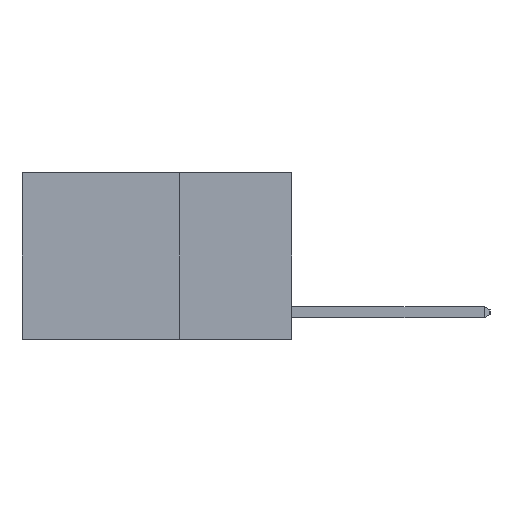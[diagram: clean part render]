
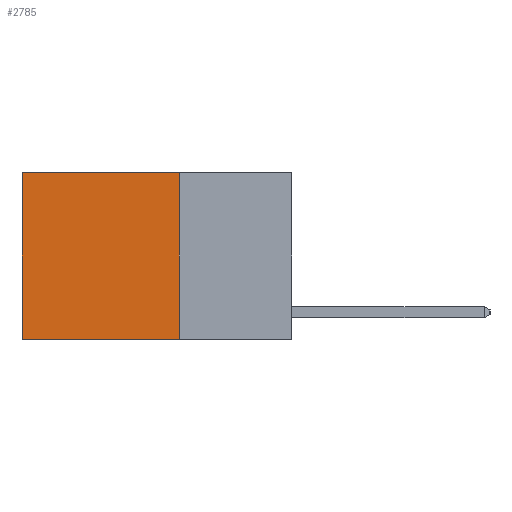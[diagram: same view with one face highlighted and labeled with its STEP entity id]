
A CAD part, left-side view. The second image highlights one B-rep face of the part: STEP entity #2785.
In plain terms, the highlighted planar face has unit normal (-1, 0, 0).
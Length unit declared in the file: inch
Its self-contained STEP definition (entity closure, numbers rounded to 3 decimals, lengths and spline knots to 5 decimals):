
#176 = EDGE_CURVE ( 'NONE', #11325, #1488, #7365, .T. ) ;
#325 = CARTESIAN_POINT ( 'NONE',  ( 0.2625, 0.25, -0.37 ) ) ;
#574 = EDGE_LOOP ( 'NONE', ( #7334, #2866, #12670, #5633 ) ) ;
#580 = EDGE_CURVE ( 'NONE', #3494, #11325, #13664, .T. ) ;
#937 = DIRECTION ( 'NONE',  ( 0., 1., 0. ) ) ;
#1488 = VERTEX_POINT ( 'NONE', #12290 ) ;
#2056 = VERTEX_POINT ( 'NONE', #325 ) ;
#2294 = DIRECTION ( 'NONE',  ( 0., 0., -1. ) ) ;
#2459 = LINE ( 'NONE', #8184, #11899 ) ;
#2785 = ADVANCED_FACE ( 'NONE', ( #12186 ), #4285, .F. ) ;
#2866 = ORIENTED_EDGE ( 'NONE', *, *, #13939, .F. ) ;
#3155 = CARTESIAN_POINT ( 'NONE',  ( 0.2625, 0.6, 0. ) ) ;
#3494 = VERTEX_POINT ( 'NONE', #13856 ) ;
#3733 = CARTESIAN_POINT ( 'NONE',  ( 0.2625, 0.25, 0. ) ) ;
#4285 = PLANE ( 'NONE',  #13534 ) ;
#5207 = DIRECTION ( 'NONE',  ( 0., 0., -1. ) ) ;
#5462 = CARTESIAN_POINT ( 'NONE',  ( 0.2625, 0.25, 0. ) ) ;
#5633 = ORIENTED_EDGE ( 'NONE', *, *, #580, .T. ) ;
#6418 = VECTOR ( 'NONE', #11287, 39.37008 ) ;
#6663 = DIRECTION ( 'NONE',  ( 0., 0., -1. ) ) ;
#7334 = ORIENTED_EDGE ( 'NONE', *, *, #176, .T. ) ;
#7365 = LINE ( 'NONE', #11049, #10185 ) ;
#8184 = CARTESIAN_POINT ( 'NONE',  ( 0.2625, 0.25, 0. ) ) ;
#8997 = DIRECTION ( 'NONE',  ( 1., 0., 0. ) ) ;
#9219 = LINE ( 'NONE', #11333, #6418 ) ;
#10185 = VECTOR ( 'NONE', #5207, 39.37008 ) ;
#11049 = CARTESIAN_POINT ( 'NONE',  ( 0.2625, 0.6, 0. ) ) ;
#11287 = DIRECTION ( 'NONE',  ( 0., 1., 0. ) ) ;
#11325 = VERTEX_POINT ( 'NONE', #3155 ) ;
#11333 = CARTESIAN_POINT ( 'NONE',  ( 0.2625, 0.25, -0.37 ) ) ;
#11899 = VECTOR ( 'NONE', #2294, 39.37008 ) ;
#12138 = EDGE_CURVE ( 'NONE', #3494, #2056, #2459, .T. ) ;
#12186 = FACE_OUTER_BOUND ( 'NONE', #574, .T. ) ;
#12290 = CARTESIAN_POINT ( 'NONE',  ( 0.2625, 0.6, -0.37 ) ) ;
#12670 = ORIENTED_EDGE ( 'NONE', *, *, #12138, .F. ) ;
#13290 = VECTOR ( 'NONE', #937, 39.37008 ) ;
#13534 = AXIS2_PLACEMENT_3D ( 'NONE', #5462, #8997, #6663 ) ;
#13664 = LINE ( 'NONE', #3733, #13290 ) ;
#13856 = CARTESIAN_POINT ( 'NONE',  ( 0.2625, 0.25, 0. ) ) ;
#13939 = EDGE_CURVE ( 'NONE', #2056, #1488, #9219, .T. ) ;
